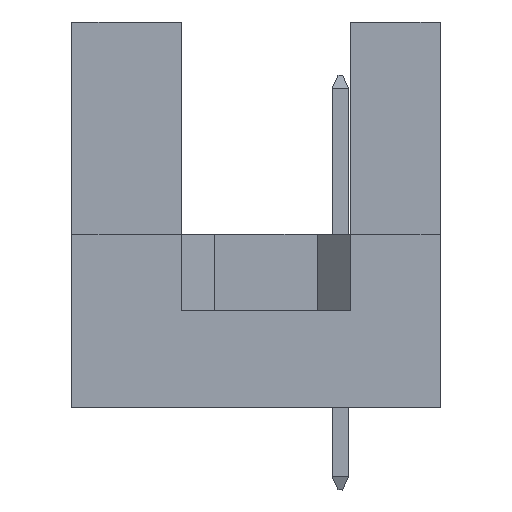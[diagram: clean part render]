
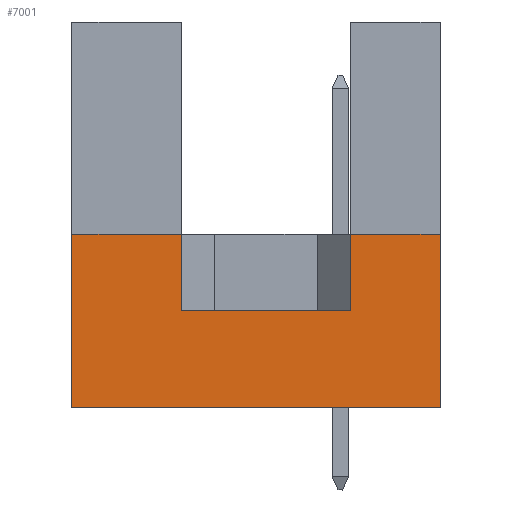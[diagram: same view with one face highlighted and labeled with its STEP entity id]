
A CAD part, left-side view. The second image highlights one B-rep face of the part: STEP entity #7001.
In plain terms, the highlighted planar face has unit normal (-1, 0, 0).
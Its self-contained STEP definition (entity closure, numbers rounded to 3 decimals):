
#179 = CARTESIAN_POINT ( 'NONE',  ( -27.5, 0., 5.2 ) ) ;
#491 = ORIENTED_EDGE ( 'NONE', *, *, #8484, .F. ) ;
#588 = CARTESIAN_POINT ( 'NONE',  ( -27.5, 11.1, 0. ) ) ;
#724 = ORIENTED_EDGE ( 'NONE', *, *, #3151, .F. ) ;
#818 = ORIENTED_EDGE ( 'NONE', *, *, #8592, .F. ) ;
#944 = VERTEX_POINT ( 'NONE', #1477 ) ;
#1165 = DIRECTION ( 'NONE',  ( 0., -1., 0. ) ) ;
#1411 = CARTESIAN_POINT ( 'NONE',  ( -27.5, 2.71, 2.9 ) ) ;
#1477 = CARTESIAN_POINT ( 'NONE',  ( -27.5, 7.79, 5.2 ) ) ;
#1566 = VERTEX_POINT ( 'NONE', #5605 ) ;
#1606 = DIRECTION ( 'NONE',  ( 0., 0., 1. ) ) ;
#1690 = CARTESIAN_POINT ( 'NONE',  ( -27.5, 11.1, 5.2 ) ) ;
#1859 = CARTESIAN_POINT ( 'NONE',  ( -27.5, 7.79, 2.9 ) ) ;
#1990 = LINE ( 'NONE', #4148, #5508 ) ;
#2015 = DIRECTION ( 'NONE',  ( 0., 0., -1. ) ) ;
#2138 = VECTOR ( 'NONE', #8538, 1000. ) ;
#2155 = CARTESIAN_POINT ( 'NONE',  ( -27.5, 2.71, 2.9 ) ) ;
#2308 = CARTESIAN_POINT ( 'NONE',  ( -27.5, 11.1, 5.2 ) ) ;
#2483 = LINE ( 'NONE', #1859, #6858 ) ;
#2585 = CARTESIAN_POINT ( 'NONE',  ( -27.5, 11.1, 5.2 ) ) ;
#2720 = DIRECTION ( 'NONE',  ( 1., 0., 0. ) ) ;
#2841 = VERTEX_POINT ( 'NONE', #6692 ) ;
#2941 = AXIS2_PLACEMENT_3D ( 'NONE', #7239, #2720, #2015 ) ;
#2964 = VECTOR ( 'NONE', #3322, 1000. ) ;
#2967 = CARTESIAN_POINT ( 'NONE',  ( -27.5, 0., 0. ) ) ;
#3033 = ORIENTED_EDGE ( 'NONE', *, *, #9062, .F. ) ;
#3063 = EDGE_CURVE ( 'NONE', #3203, #944, #8582, .T. ) ;
#3151 = EDGE_CURVE ( 'NONE', #3985, #1566, #8626, .T. ) ;
#3203 = VERTEX_POINT ( 'NONE', #4651 ) ;
#3322 = DIRECTION ( 'NONE',  ( 0., -1., 0. ) ) ;
#3501 = EDGE_CURVE ( 'NONE', #7793, #5442, #3637, .T. ) ;
#3637 = LINE ( 'NONE', #588, #8466 ) ;
#3655 = LINE ( 'NONE', #2967, #4144 ) ;
#3665 = ORIENTED_EDGE ( 'NONE', *, *, #9207, .T. ) ;
#3985 = VERTEX_POINT ( 'NONE', #1411 ) ;
#4144 = VECTOR ( 'NONE', #1606, 1000. ) ;
#4148 = CARTESIAN_POINT ( 'NONE',  ( -27.5, 11.1, 0. ) ) ;
#4355 = FACE_OUTER_BOUND ( 'NONE', #4477, .T. ) ;
#4414 = DIRECTION ( 'NONE',  ( 0., -1., 0. ) ) ;
#4446 = VECTOR ( 'NONE', #4414, 1000. ) ;
#4474 = LINE ( 'NONE', #2308, #4446 ) ;
#4477 = EDGE_LOOP ( 'NONE', ( #3033, #6344, #818, #9302, #3665, #8429, #491, #724 ) ) ;
#4651 = CARTESIAN_POINT ( 'NONE',  ( -27.5, 7.79, 2.9 ) ) ;
#5029 = DIRECTION ( 'NONE',  ( 0., 0., 1. ) ) ;
#5309 = LINE ( 'NONE', #2585, #2964 ) ;
#5442 = VERTEX_POINT ( 'NONE', #1690 ) ;
#5508 = VECTOR ( 'NONE', #7746, 1000. ) ;
#5605 = CARTESIAN_POINT ( 'NONE',  ( -27.5, 2.71, 5.2 ) ) ;
#5642 = DIRECTION ( 'NONE',  ( 0., 0., 1. ) ) ;
#5826 = VERTEX_POINT ( 'NONE', #179 ) ;
#6344 = ORIENTED_EDGE ( 'NONE', *, *, #3063, .T. ) ;
#6658 = VECTOR ( 'NONE', #5029, 1000. ) ;
#6692 = CARTESIAN_POINT ( 'NONE',  ( -27.5, 0., 0. ) ) ;
#6858 = VECTOR ( 'NONE', #1165, 1000. ) ;
#7001 = ADVANCED_FACE ( 'NONE', ( #4355 ), #9191, .F. ) ;
#7122 = CARTESIAN_POINT ( 'NONE',  ( -27.5, 11.1, 0. ) ) ;
#7150 = CARTESIAN_POINT ( 'NONE',  ( -27.5, 7.79, 2.9 ) ) ;
#7239 = CARTESIAN_POINT ( 'NONE',  ( -27.5, 11.1, 0. ) ) ;
#7746 = DIRECTION ( 'NONE',  ( 0., -1., 0. ) ) ;
#7793 = VERTEX_POINT ( 'NONE', #7122 ) ;
#8429 = ORIENTED_EDGE ( 'NONE', *, *, #8479, .T. ) ;
#8466 = VECTOR ( 'NONE', #5642, 1000. ) ;
#8479 = EDGE_CURVE ( 'NONE', #2841, #5826, #3655, .T. ) ;
#8484 = EDGE_CURVE ( 'NONE', #1566, #5826, #4474, .T. ) ;
#8538 = DIRECTION ( 'NONE',  ( 0., 0., 1. ) ) ;
#8582 = LINE ( 'NONE', #7150, #2138 ) ;
#8592 = EDGE_CURVE ( 'NONE', #5442, #944, #5309, .T. ) ;
#8626 = LINE ( 'NONE', #2155, #6658 ) ;
#9062 = EDGE_CURVE ( 'NONE', #3203, #3985, #2483, .T. ) ;
#9191 = PLANE ( 'NONE',  #2941 ) ;
#9207 = EDGE_CURVE ( 'NONE', #7793, #2841, #1990, .T. ) ;
#9302 = ORIENTED_EDGE ( 'NONE', *, *, #3501, .F. ) ;
